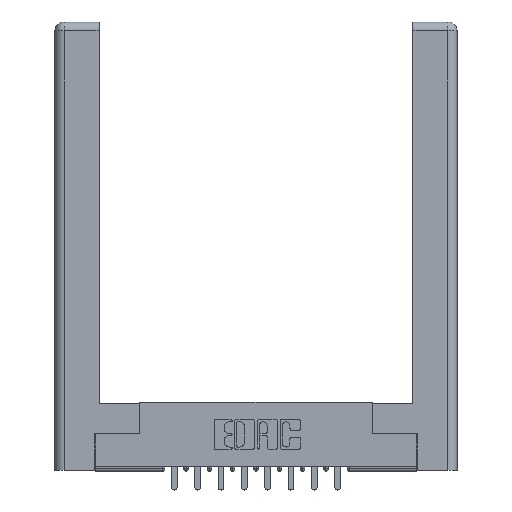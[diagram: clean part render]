
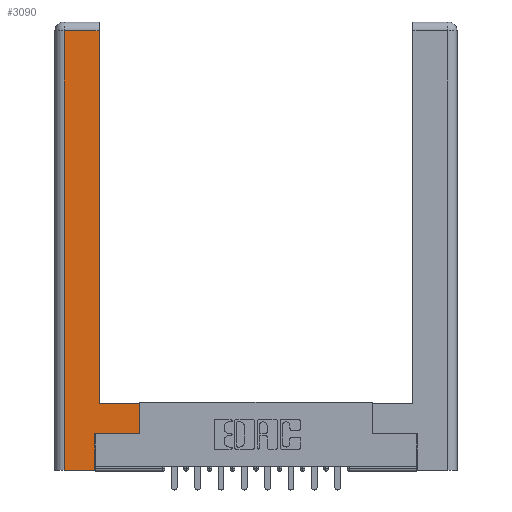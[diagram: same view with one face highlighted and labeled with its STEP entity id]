
A CAD part, top view. The second image highlights one B-rep face of the part: STEP entity #3090.
In plain terms, the highlighted planar face has unit normal (0, 0, 1).
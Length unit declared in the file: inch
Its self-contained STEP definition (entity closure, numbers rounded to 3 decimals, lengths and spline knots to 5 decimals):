
#99 = DIRECTION ( 'NONE',  ( -1., 0., 0. ) ) ;
#215 = CARTESIAN_POINT ( 'NONE',  ( 0.295, 2.94, 0. ) ) ;
#390 = CARTESIAN_POINT ( 'NONE',  ( 0.265, 0.245, 0. ) ) ;
#485 = DIRECTION ( 'NONE',  ( 1., 0., 0. ) ) ;
#573 = DIRECTION ( 'NONE',  ( 0., 1., 0. ) ) ;
#935 = DIRECTION ( 'NONE',  ( -1., 0., 0. ) ) ;
#1384 = LINE ( 'NONE', #5882, #3839 ) ;
#1429 = VERTEX_POINT ( 'NONE', #6861 ) ;
#1481 = VERTEX_POINT ( 'NONE', #7693 ) ;
#1504 = CARTESIAN_POINT ( 'NONE',  ( 0.0615, 2.94, 0. ) ) ;
#1646 = ORIENTED_EDGE ( 'NONE', *, *, #12822, .T. ) ;
#1792 = CARTESIAN_POINT ( 'NONE',  ( 0.265, 0., 0. ) ) ;
#2514 = EDGE_CURVE ( 'NONE', #4128, #1429, #10143, .T. ) ;
#2700 = EDGE_LOOP ( 'NONE', ( #9620, #4389, #5126, #4608, #13301, #6663, #1646, #12795 ) ) ;
#3090 = ADVANCED_FACE ( 'NONE', ( #5454 ), #11318, .F. ) ;
#3341 = EDGE_CURVE ( 'NONE', #9942, #1481, #11590, .T. ) ;
#3443 = CARTESIAN_POINT ( 'NONE',  ( 0.0615, 0., 0. ) ) ;
#3516 = VERTEX_POINT ( 'NONE', #13441 ) ;
#3712 = DIRECTION ( 'NONE',  ( 0., 1., 0. ) ) ;
#3839 = VECTOR ( 'NONE', #573, 39.37008 ) ;
#4128 = VERTEX_POINT ( 'NONE', #1504 ) ;
#4389 = ORIENTED_EDGE ( 'NONE', *, *, #4937, .T. ) ;
#4608 = ORIENTED_EDGE ( 'NONE', *, *, #11739, .T. ) ;
#4707 = LINE ( 'NONE', #5737, #14145 ) ;
#4796 = DIRECTION ( 'NONE',  ( -1., 0., 0. ) ) ;
#4937 = EDGE_CURVE ( 'NONE', #5045, #4128, #6519, .T. ) ;
#5045 = VERTEX_POINT ( 'NONE', #215 ) ;
#5126 = ORIENTED_EDGE ( 'NONE', *, *, #2514, .T. ) ;
#5454 = FACE_OUTER_BOUND ( 'NONE', #2700, .T. ) ;
#5737 = CARTESIAN_POINT ( 'NONE',  ( 0.295, 3., 0. ) ) ;
#5882 = CARTESIAN_POINT ( 'NONE',  ( 0.565, 0.45, 0. ) ) ;
#6319 = VECTOR ( 'NONE', #935, 39.37008 ) ;
#6519 = LINE ( 'NONE', #10994, #6319 ) ;
#6648 = VECTOR ( 'NONE', #485, 39.37008 ) ;
#6663 = ORIENTED_EDGE ( 'NONE', *, *, #13323, .T. ) ;
#6861 = CARTESIAN_POINT ( 'NONE',  ( 0.0615, 0., 0. ) ) ;
#7128 = VECTOR ( 'NONE', #12211, 39.37008 ) ;
#7693 = CARTESIAN_POINT ( 'NONE',  ( 0.295, 0.45, 0. ) ) ;
#9009 = LINE ( 'NONE', #10033, #7128 ) ;
#9385 = LINE ( 'NONE', #13832, #10088 ) ;
#9490 = VECTOR ( 'NONE', #10767, 39.37008 ) ;
#9620 = ORIENTED_EDGE ( 'NONE', *, *, #14348, .T. ) ;
#9942 = VERTEX_POINT ( 'NONE', #10692 ) ;
#9963 = VERTEX_POINT ( 'NONE', #1792 ) ;
#10033 = CARTESIAN_POINT ( 'NONE',  ( 0.265, 0., 0. ) ) ;
#10088 = VECTOR ( 'NONE', #3712, 39.37008 ) ;
#10143 = LINE ( 'NONE', #3443, #9490 ) ;
#10544 = CARTESIAN_POINT ( 'NONE',  ( 0.565, 0.245, 0. ) ) ;
#10692 = CARTESIAN_POINT ( 'NONE',  ( 0.565, 0.45, 0. ) ) ;
#10696 = LINE ( 'NONE', #10544, #6648 ) ;
#10767 = DIRECTION ( 'NONE',  ( 0., -1., 0. ) ) ;
#10994 = CARTESIAN_POINT ( 'NONE',  ( 0.0615, 2.94, 0. ) ) ;
#11027 = DIRECTION ( 'NONE',  ( 0., 0., -1. ) ) ;
#11064 = EDGE_CURVE ( 'NONE', #9963, #11914, #9385, .T. ) ;
#11318 = PLANE ( 'NONE',  #13306 ) ;
#11371 = DIRECTION ( 'NONE',  ( 0., 1., 0. ) ) ;
#11590 = LINE ( 'NONE', #12777, #13761 ) ;
#11739 = EDGE_CURVE ( 'NONE', #1429, #9963, #9009, .T. ) ;
#11914 = VERTEX_POINT ( 'NONE', #390 ) ;
#12198 = CARTESIAN_POINT ( 'NONE',  ( 0., 0., 0. ) ) ;
#12211 = DIRECTION ( 'NONE',  ( 1., 0., 0. ) ) ;
#12777 = CARTESIAN_POINT ( 'NONE',  ( 0.295, 0.45, 0. ) ) ;
#12795 = ORIENTED_EDGE ( 'NONE', *, *, #3341, .T. ) ;
#12822 = EDGE_CURVE ( 'NONE', #3516, #9942, #1384, .T. ) ;
#13301 = ORIENTED_EDGE ( 'NONE', *, *, #11064, .T. ) ;
#13306 = AXIS2_PLACEMENT_3D ( 'NONE', #12198, #11027, #99 ) ;
#13323 = EDGE_CURVE ( 'NONE', #11914, #3516, #10696, .T. ) ;
#13441 = CARTESIAN_POINT ( 'NONE',  ( 0.565, 0.245, 0. ) ) ;
#13761 = VECTOR ( 'NONE', #4796, 39.37008 ) ;
#13832 = CARTESIAN_POINT ( 'NONE',  ( 0.265, 0.245, 0. ) ) ;
#14145 = VECTOR ( 'NONE', #11371, 39.37008 ) ;
#14348 = EDGE_CURVE ( 'NONE', #1481, #5045, #4707, .T. ) ;
